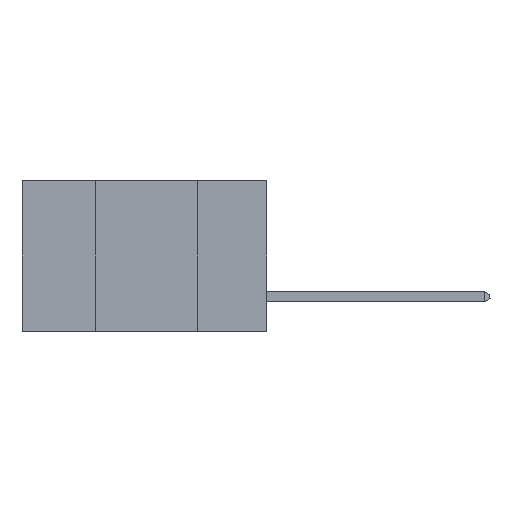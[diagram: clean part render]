
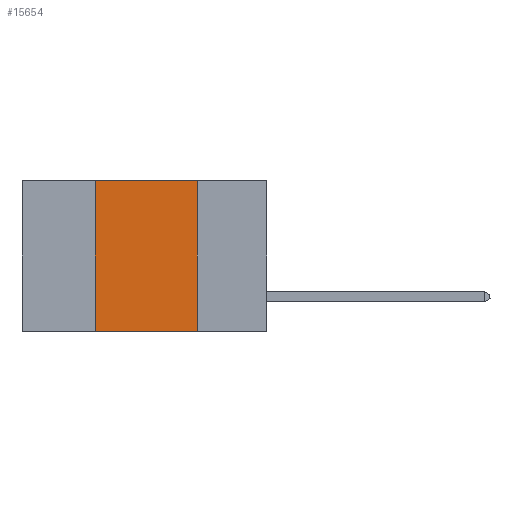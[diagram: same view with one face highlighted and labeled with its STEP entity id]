
A CAD part, left-side view. The second image highlights one B-rep face of the part: STEP entity #15654.
In plain terms, the highlighted planar face has unit normal (-1, 0, 0).
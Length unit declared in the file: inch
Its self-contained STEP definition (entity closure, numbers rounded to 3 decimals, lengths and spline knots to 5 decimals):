
#330 = CARTESIAN_POINT ( 'NONE',  ( 0., 0.17, -0.37 ) ) ;
#489 = ORIENTED_EDGE ( 'NONE', *, *, #11839, .T. ) ;
#652 = VECTOR ( 'NONE', #12675, 39.37008 ) ;
#1232 = EDGE_CURVE ( 'NONE', #19009, #18471, #16565, .T. ) ;
#2136 = DIRECTION ( 'NONE',  ( 0., 0., -1. ) ) ;
#2295 = CARTESIAN_POINT ( 'NONE',  ( 0., 0.6, -0.37 ) ) ;
#3619 = EDGE_CURVE ( 'NONE', #5879, #3776, #9271, .T. ) ;
#3776 = VERTEX_POINT ( 'NONE', #18575 ) ;
#4322 = LINE ( 'NONE', #10816, #5079 ) ;
#5079 = VECTOR ( 'NONE', #12548, 39.37008 ) ;
#5879 = VERTEX_POINT ( 'NONE', #20847 ) ;
#5995 = EDGE_CURVE ( 'NONE', #3776, #19009, #4322, .T. ) ;
#6220 = FACE_OUTER_BOUND ( 'NONE', #13979, .T. ) ;
#6679 = CARTESIAN_POINT ( 'NONE',  ( 0., 0.17, 0. ) ) ;
#7254 = CARTESIAN_POINT ( 'NONE',  ( 0., 0.6, 0. ) ) ;
#8224 = ORIENTED_EDGE ( 'NONE', *, *, #1232, .F. ) ;
#9013 = ORIENTED_EDGE ( 'NONE', *, *, #5995, .F. ) ;
#9271 = LINE ( 'NONE', #11151, #14914 ) ;
#10816 = CARTESIAN_POINT ( 'NONE',  ( 0., 0.6, 0. ) ) ;
#11025 = CARTESIAN_POINT ( 'NONE',  ( 0., 0.17, 0. ) ) ;
#11151 = CARTESIAN_POINT ( 'NONE',  ( 0., 0.42, 0. ) ) ;
#11297 = AXIS2_PLACEMENT_3D ( 'NONE', #7254, #18710, #2136 ) ;
#11839 = EDGE_CURVE ( 'NONE', #5879, #18471, #13656, .T. ) ;
#12548 = DIRECTION ( 'NONE',  ( 0., -1., 0. ) ) ;
#12675 = DIRECTION ( 'NONE',  ( 0., 0., -1. ) ) ;
#13656 = LINE ( 'NONE', #2295, #19552 ) ;
#13753 = PLANE ( 'NONE',  #11297 ) ;
#13979 = EDGE_LOOP ( 'NONE', ( #8224, #9013, #17323, #489 ) ) ;
#14914 = VECTOR ( 'NONE', #21104, 39.37008 ) ;
#15654 = ADVANCED_FACE ( 'NONE', ( #6220 ), #13753, .F. ) ;
#16565 = LINE ( 'NONE', #11025, #652 ) ;
#17028 = DIRECTION ( 'NONE',  ( 0., -1., 0. ) ) ;
#17323 = ORIENTED_EDGE ( 'NONE', *, *, #3619, .F. ) ;
#18471 = VERTEX_POINT ( 'NONE', #330 ) ;
#18575 = CARTESIAN_POINT ( 'NONE',  ( 0., 0.42, 0. ) ) ;
#18710 = DIRECTION ( 'NONE',  ( 1., 0., 0. ) ) ;
#19009 = VERTEX_POINT ( 'NONE', #6679 ) ;
#19552 = VECTOR ( 'NONE', #17028, 39.37008 ) ;
#20847 = CARTESIAN_POINT ( 'NONE',  ( 0., 0.42, -0.37 ) ) ;
#21104 = DIRECTION ( 'NONE',  ( 0., 0., 1. ) ) ;
